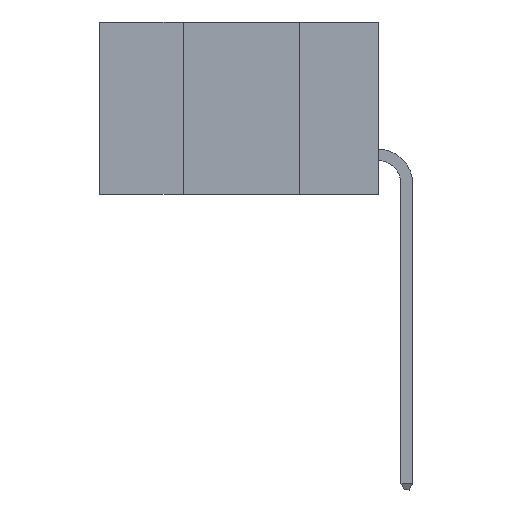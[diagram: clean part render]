
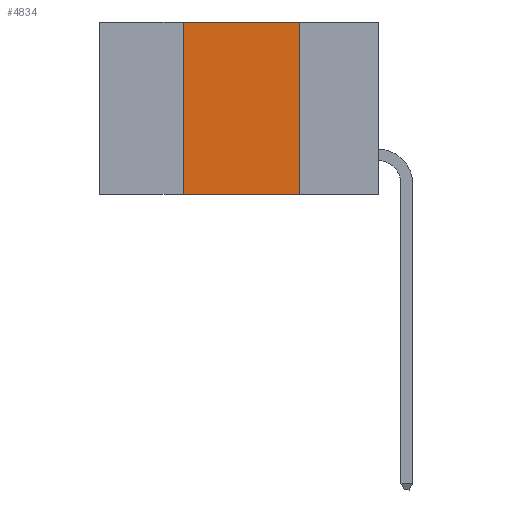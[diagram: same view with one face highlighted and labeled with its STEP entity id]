
A CAD part, left-side view. The second image highlights one B-rep face of the part: STEP entity #4834.
In plain terms, the highlighted planar face has unit normal (-1, 0, 0).
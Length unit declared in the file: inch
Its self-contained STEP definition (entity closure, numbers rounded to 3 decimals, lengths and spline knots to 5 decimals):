
#909 = LINE ( 'NONE', #25437, #24004 ) ;
#938 = VECTOR ( 'NONE', #18170, 39.37008 ) ;
#3055 = DIRECTION ( 'NONE',  ( 0., -1., 0. ) ) ;
#4661 = AXIS2_PLACEMENT_3D ( 'NONE', #28404, #9028, #13341 ) ;
#4834 = ADVANCED_FACE ( 'NONE', ( #12985 ), #13234, .F. ) ;
#4900 = ORIENTED_EDGE ( 'NONE', *, *, #23496, .F. ) ;
#7157 = CARTESIAN_POINT ( 'NONE',  ( 0., 0.6, -0.37 ) ) ;
#8280 = ORIENTED_EDGE ( 'NONE', *, *, #10646, .F. ) ;
#9028 = DIRECTION ( 'NONE',  ( 1., 0., 0. ) ) ;
#10646 = EDGE_CURVE ( 'NONE', #23255, #11843, #19837, .T. ) ;
#10865 = CARTESIAN_POINT ( 'NONE',  ( 0., 0.42, 0. ) ) ;
#11254 = VERTEX_POINT ( 'NONE', #17752 ) ;
#11306 = CARTESIAN_POINT ( 'NONE',  ( 0., 0.42, 0. ) ) ;
#11482 = EDGE_CURVE ( 'NONE', #23255, #11254, #19105, .T. ) ;
#11843 = VERTEX_POINT ( 'NONE', #10865 ) ;
#12132 = DIRECTION ( 'NONE',  ( 0., -1., 0. ) ) ;
#12266 = LINE ( 'NONE', #28730, #23473 ) ;
#12985 = FACE_OUTER_BOUND ( 'NONE', #21206, .T. ) ;
#13234 = PLANE ( 'NONE',  #4661 ) ;
#13341 = DIRECTION ( 'NONE',  ( 0., 0., -1. ) ) ;
#14532 = ORIENTED_EDGE ( 'NONE', *, *, #28504, .F. ) ;
#17752 = CARTESIAN_POINT ( 'NONE',  ( 0., 0.17, -0.37 ) ) ;
#18170 = DIRECTION ( 'NONE',  ( 0., 0., 1. ) ) ;
#19105 = LINE ( 'NONE', #7157, #20812 ) ;
#19837 = LINE ( 'NONE', #11306, #938 ) ;
#20812 = VECTOR ( 'NONE', #12132, 39.37008 ) ;
#21206 = EDGE_LOOP ( 'NONE', ( #14532, #4900, #8280, #22465 ) ) ;
#21394 = CARTESIAN_POINT ( 'NONE',  ( 0., 0.17, 0. ) ) ;
#22465 = ORIENTED_EDGE ( 'NONE', *, *, #11482, .T. ) ;
#23255 = VERTEX_POINT ( 'NONE', #24788 ) ;
#23473 = VECTOR ( 'NONE', #24412, 39.37008 ) ;
#23496 = EDGE_CURVE ( 'NONE', #11843, #25513, #909, .T. ) ;
#24004 = VECTOR ( 'NONE', #3055, 39.37008 ) ;
#24412 = DIRECTION ( 'NONE',  ( 0., 0., -1. ) ) ;
#24788 = CARTESIAN_POINT ( 'NONE',  ( 0., 0.42, -0.37 ) ) ;
#25437 = CARTESIAN_POINT ( 'NONE',  ( 0., 0.6, 0. ) ) ;
#25513 = VERTEX_POINT ( 'NONE', #21394 ) ;
#28404 = CARTESIAN_POINT ( 'NONE',  ( 0., 0.6, 0. ) ) ;
#28504 = EDGE_CURVE ( 'NONE', #25513, #11254, #12266, .T. ) ;
#28730 = CARTESIAN_POINT ( 'NONE',  ( 0., 0.17, 0. ) ) ;
